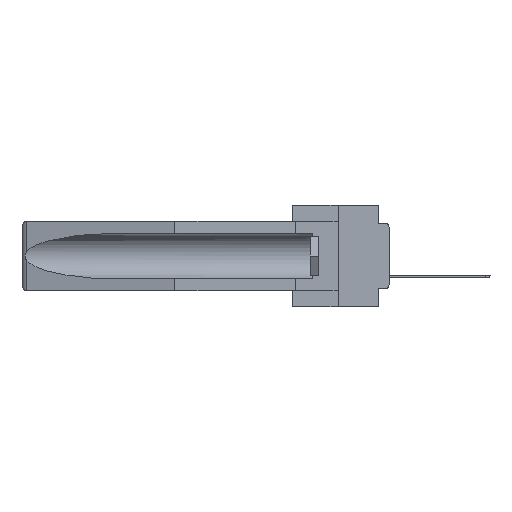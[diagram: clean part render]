
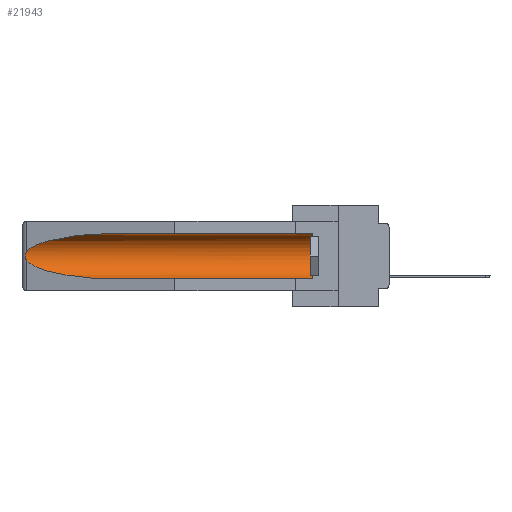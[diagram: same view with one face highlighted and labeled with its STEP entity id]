
A CAD part, left-side view. The second image highlights one B-rep face of the part: STEP entity #21943.
In plain terms, the highlighted cylindrical face has radius 2.857 mm (diameter 5.715 mm), a partial arc.
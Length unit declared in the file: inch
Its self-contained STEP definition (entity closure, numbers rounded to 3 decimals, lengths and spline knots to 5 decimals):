
#1059 = CARTESIAN_POINT ( 'NONE',  ( 0.155, 1.07973, -0.059 ) ) ;
#1297 = CARTESIAN_POINT ( 'NONE',  ( 0.155, 1.07973, -0.284 ) ) ;
#1437 = CARTESIAN_POINT ( 'NONE',  ( 0.2673, 1.53269, -0.17917 ) ) ;
#1959 = CARTESIAN_POINT ( 'NONE',  ( 0.26537, 1.52718, -0.19328 ) ) ;
#2134 = CARTESIAN_POINT ( 'NONE',  ( 0.26537, 1.52718, -0.14972 ) ) ;
#3159 = EDGE_CURVE ( 'NONE', #20523, #18067, #7605, .T. ) ;
#3355 = CARTESIAN_POINT ( 'NONE',  ( 0.2675, 1.53308, -0.16763 ) ) ;
#3595 = CARTESIAN_POINT ( 'NONE',  ( 0.2673, 1.5327, -0.16383 ) ) ;
#4067 = CARTESIAN_POINT ( 'NONE',  ( 0.26537, 1.52718, -0.19328 ) ) ;
#5049 = ORIENTED_EDGE ( 'NONE', *, *, #35166, .T. ) ;
#5235 = ORIENTED_EDGE ( 'NONE', *, *, #6788, .F. ) ;
#5270 = CARTESIAN_POINT ( 'NONE',  ( 0.155, -0.30754, -0.1715 ) ) ;
#5402 =( BOUNDED_CURVE ( )  B_SPLINE_CURVE ( 3, ( #4067, #23258, #20157, #1297 ),
 .UNSPECIFIED., .F., .F. ) 
 B_SPLINE_CURVE_WITH_KNOTS ( ( 4, 4 ),
 ( 0.1948, 1.5708 ),
 .UNSPECIFIED. ) 
 CURVE ( )  GEOMETRIC_REPRESENTATION_ITEM ( )  RATIONAL_B_SPLINE_CURVE ( ( 1., 0.848, 0.848, 1. ) ) 
 REPRESENTATION_ITEM ( '' )  );
#6788 = EDGE_CURVE ( 'NONE', #8666, #15193, #27478, .T. ) ;
#7389 = AXIS2_PLACEMENT_3D ( 'NONE', #7399, #16417, #24608 ) ;
#7399 = CARTESIAN_POINT ( 'NONE',  ( 0.155, 0.126, -0.1715 ) ) ;
#7605 =( BOUNDED_CURVE ( )  B_SPLINE_CURVE ( 3, ( #33397, #28440, #22434, #22791 ),
 .UNSPECIFIED., .F., .F. ) 
 B_SPLINE_CURVE_WITH_KNOTS ( ( 4, 4 ),
 ( 4.71239, 6.08839 ),
 .UNSPECIFIED. ) 
 CURVE ( )  GEOMETRIC_REPRESENTATION_ITEM ( )  RATIONAL_B_SPLINE_CURVE ( ( 1., 0.848, 0.848, 1. ) ) 
 REPRESENTATION_ITEM ( '' )  );
#7799 = DIRECTION ( 'NONE',  ( 0., 0., 1. ) ) ;
#8207 = CIRCLE ( 'NONE', #7389, 0.1125 ) ;
#8666 = VERTEX_POINT ( 'NONE', #21972 ) ;
#10953 = EDGE_CURVE ( 'NONE', #26408, #20523, #25731, .T. ) ;
#11726 = ORIENTED_EDGE ( 'NONE', *, *, #10953, .T. ) ;
#11761 = B_SPLINE_CURVE_WITH_KNOTS ( 'NONE', 3,
 ( #31038, #27963, #17260, #3595, #3355, #17868, #1437, #34362, #31638, #34120 ),
 .UNSPECIFIED., .F., .F.,
 ( 4, 2, 2, 2, 4 ),
 ( 0., 0.00029, 0.00058, 0.00087, 0.00117 ),
 .UNSPECIFIED. ) ;
#11795 = DIRECTION ( 'NONE',  ( 0., 1., 0. ) ) ;
#12045 = CARTESIAN_POINT ( 'NONE',  ( 0.155, -0.30754, -0.284 ) ) ;
#12764 = DIRECTION ( 'NONE',  ( 0., 1., 0. ) ) ;
#13124 = FACE_OUTER_BOUND ( 'NONE', #23250, .T. ) ;
#15193 = VERTEX_POINT ( 'NONE', #16118 ) ;
#16118 = CARTESIAN_POINT ( 'NONE',  ( 0.155, 1.07973, -0.284 ) ) ;
#16332 = DIRECTION ( 'NONE',  ( 0., 1., 0. ) ) ;
#16417 = DIRECTION ( 'NONE',  ( 0., -1., 0. ) ) ;
#17118 = VECTOR ( 'NONE', #11795, 39.37008 ) ;
#17260 = CARTESIAN_POINT ( 'NONE',  ( 0.26654, 1.53092, -0.15636 ) ) ;
#17868 = CARTESIAN_POINT ( 'NONE',  ( 0.2675, 1.53308, -0.17534 ) ) ;
#18067 = VERTEX_POINT ( 'NONE', #2134 ) ;
#20157 = CARTESIAN_POINT ( 'NONE',  ( 0.21114, 1.30732, -0.284 ) ) ;
#20484 = EDGE_CURVE ( 'NONE', #26461, #15193, #5402, .T. ) ;
#20523 = VERTEX_POINT ( 'NONE', #1059 ) ;
#21028 = VECTOR ( 'NONE', #12764, 39.37008 ) ;
#21943 = ADVANCED_FACE ( 'NONE', ( #13124 ), #26042, .F. ) ;
#21972 = CARTESIAN_POINT ( 'NONE',  ( 0.155, 0.126, -0.284 ) ) ;
#22434 = CARTESIAN_POINT ( 'NONE',  ( 0.25451, 1.48313, -0.09465 ) ) ;
#22791 = CARTESIAN_POINT ( 'NONE',  ( 0.26537, 1.52718, -0.14972 ) ) ;
#23250 = EDGE_LOOP ( 'NONE', ( #26384, #5049, #32710, #5235, #23709, #11726 ) ) ;
#23258 = CARTESIAN_POINT ( 'NONE',  ( 0.25451, 1.48313, -0.24835 ) ) ;
#23709 = ORIENTED_EDGE ( 'NONE', *, *, #32408, .T. ) ;
#24063 = CARTESIAN_POINT ( 'NONE',  ( 0.155, 0.126, -0.059 ) ) ;
#24608 = DIRECTION ( 'NONE',  ( 0., 0., 1. ) ) ;
#25731 = LINE ( 'NONE', #26710, #21028 ) ;
#26042 = CYLINDRICAL_SURFACE ( 'NONE', #26515, 0.1125 ) ;
#26384 = ORIENTED_EDGE ( 'NONE', *, *, #3159, .T. ) ;
#26408 = VERTEX_POINT ( 'NONE', #24063 ) ;
#26461 = VERTEX_POINT ( 'NONE', #1959 ) ;
#26515 = AXIS2_PLACEMENT_3D ( 'NONE', #5270, #16332, #7799 ) ;
#26710 = CARTESIAN_POINT ( 'NONE',  ( 0.155, -0.30754, -0.059 ) ) ;
#27478 = LINE ( 'NONE', #12045, #17118 ) ;
#27963 = CARTESIAN_POINT ( 'NONE',  ( 0.26597, 1.52961, -0.15275 ) ) ;
#28440 = CARTESIAN_POINT ( 'NONE',  ( 0.21114, 1.30732, -0.059 ) ) ;
#31038 = CARTESIAN_POINT ( 'NONE',  ( 0.26537, 1.52718, -0.14972 ) ) ;
#31638 = CARTESIAN_POINT ( 'NONE',  ( 0.26597, 1.5296, -0.19026 ) ) ;
#32408 = EDGE_CURVE ( 'NONE', #8666, #26408, #8207, .T. ) ;
#32710 = ORIENTED_EDGE ( 'NONE', *, *, #20484, .T. ) ;
#33397 = CARTESIAN_POINT ( 'NONE',  ( 0.155, 1.07973, -0.059 ) ) ;
#34120 = CARTESIAN_POINT ( 'NONE',  ( 0.26537, 1.52718, -0.19328 ) ) ;
#34362 = CARTESIAN_POINT ( 'NONE',  ( 0.26655, 1.53094, -0.18657 ) ) ;
#35166 = EDGE_CURVE ( 'NONE', #18067, #26461, #11761, .T. ) ;
